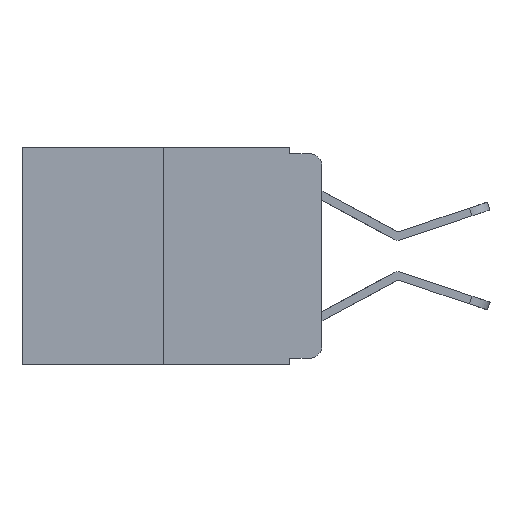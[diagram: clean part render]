
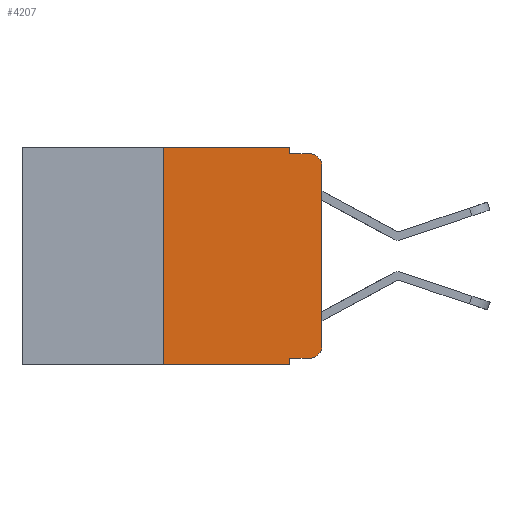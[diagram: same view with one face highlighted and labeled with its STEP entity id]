
A CAD part, left-side view. The second image highlights one B-rep face of the part: STEP entity #4207.
In plain terms, the highlighted planar face has unit normal (-1, 0, 0).
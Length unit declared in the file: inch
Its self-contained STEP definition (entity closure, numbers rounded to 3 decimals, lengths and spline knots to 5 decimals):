
#212 = LINE ( 'NONE', #8934, #7662 ) ;
#297 = EDGE_CURVE ( 'NONE', #12256, #12017, #4708, .T. ) ;
#333 = VERTEX_POINT ( 'NONE', #1383 ) ;
#402 = CARTESIAN_POINT ( 'NONE',  ( 0., 0.02, -0.01 ) ) ;
#581 = CARTESIAN_POINT ( 'NONE',  ( 0., 0.02, -0.313 ) ) ;
#636 = DIRECTION ( 'NONE',  ( 0., -1., 0. ) ) ;
#1046 = DIRECTION ( 'NONE',  ( 0., 0., 1. ) ) ;
#1383 = CARTESIAN_POINT ( 'NONE',  ( 0., 0., -0.03 ) ) ;
#1679 = EDGE_CURVE ( 'NONE', #333, #10944, #9235, .T. ) ;
#2024 = PLANE ( 'NONE',  #10068 ) ;
#2312 = CARTESIAN_POINT ( 'NONE',  ( 0., 0.051, -0.333 ) ) ;
#2978 = CARTESIAN_POINT ( 'NONE',  ( 0., 0.051, -0.01 ) ) ;
#3108 = EDGE_CURVE ( 'NONE', #14213, #8641, #9107, .T. ) ;
#3114 = ORIENTED_EDGE ( 'NONE', *, *, #12327, .T. ) ;
#3122 = DIRECTION ( 'NONE',  ( -1., 0., 0. ) ) ;
#3251 = FACE_OUTER_BOUND ( 'NONE', #3727, .T. ) ;
#3275 = DIRECTION ( 'NONE',  ( -1., 0., 0. ) ) ;
#3452 = DIRECTION ( 'NONE',  ( 0., 0., -1. ) ) ;
#3561 = CARTESIAN_POINT ( 'NONE',  ( 0., 0.051, 0. ) ) ;
#3665 = ORIENTED_EDGE ( 'NONE', *, *, #6255, .T. ) ;
#3727 = EDGE_LOOP ( 'NONE', ( #3665, #12600, #4536, #15587, #9954, #3835, #3114, #15372, #4014, #5535 ) ) ;
#3753 = VECTOR ( 'NONE', #6467, 39.37008 ) ;
#3756 = VECTOR ( 'NONE', #6733, 39.37008 ) ;
#3835 = ORIENTED_EDGE ( 'NONE', *, *, #9196, .F. ) ;
#4014 = ORIENTED_EDGE ( 'NONE', *, *, #7070, .T. ) ;
#4199 = CARTESIAN_POINT ( 'NONE',  ( 0., 0.051, -0.01 ) ) ;
#4207 = ADVANCED_FACE ( 'NONE', ( #3251 ), #2024, .F. ) ;
#4519 = DIRECTION ( 'NONE',  ( 0., 0., -1. ) ) ;
#4536 = ORIENTED_EDGE ( 'NONE', *, *, #13180, .F. ) ;
#4569 = VERTEX_POINT ( 'NONE', #14029 ) ;
#4619 = CARTESIAN_POINT ( 'NONE',  ( 0., 0.25, -0.343 ) ) ;
#4708 = LINE ( 'NONE', #14584, #7427 ) ;
#4967 = VERTEX_POINT ( 'NONE', #10466 ) ;
#5535 = ORIENTED_EDGE ( 'NONE', *, *, #10869, .T. ) ;
#5554 = CARTESIAN_POINT ( 'NONE',  ( 0., 0.473, 0. ) ) ;
#5562 = VECTOR ( 'NONE', #8640, 39.37008 ) ;
#6005 = CARTESIAN_POINT ( 'NONE',  ( 0., 0.473, -0.343 ) ) ;
#6115 = VECTOR ( 'NONE', #636, 39.37008 ) ;
#6255 = EDGE_CURVE ( 'NONE', #4569, #333, #212, .T. ) ;
#6301 = DIRECTION ( 'NONE',  ( 0., 0., -1. ) ) ;
#6404 = VECTOR ( 'NONE', #1046, 39.37008 ) ;
#6467 = DIRECTION ( 'NONE',  ( 0., -1., 0. ) ) ;
#6733 = DIRECTION ( 'NONE',  ( 0., -1., 0. ) ) ;
#7070 = EDGE_CURVE ( 'NONE', #12256, #4967, #12987, .T. ) ;
#7427 = VECTOR ( 'NONE', #3452, 39.37008 ) ;
#7662 = VECTOR ( 'NONE', #12722, 39.37008 ) ;
#8383 = LINE ( 'NONE', #6005, #5562 ) ;
#8492 = LINE ( 'NONE', #13249, #6404 ) ;
#8640 = DIRECTION ( 'NONE',  ( 0., -1., 0. ) ) ;
#8641 = VERTEX_POINT ( 'NONE', #12896 ) ;
#8934 = CARTESIAN_POINT ( 'NONE',  ( 0., 0., 0. ) ) ;
#9107 = LINE ( 'NONE', #12878, #3753 ) ;
#9196 = EDGE_CURVE ( 'NONE', #15084, #14213, #8492, .T. ) ;
#9235 = CIRCLE ( 'NONE', #10229, 0.02 ) ;
#9410 = CARTESIAN_POINT ( 'NONE',  ( 0., 0.02, -0.03 ) ) ;
#9634 = DIRECTION ( 'NONE',  ( 1., 0., 0. ) ) ;
#9954 = ORIENTED_EDGE ( 'NONE', *, *, #3108, .F. ) ;
#10068 = AXIS2_PLACEMENT_3D ( 'NONE', #5554, #9634, #10830 ) ;
#10219 = EDGE_CURVE ( 'NONE', #8641, #13550, #16103, .T. ) ;
#10229 = AXIS2_PLACEMENT_3D ( 'NONE', #9410, #3122, #15647 ) ;
#10466 = CARTESIAN_POINT ( 'NONE',  ( 0., 0.02, -0.333 ) ) ;
#10830 = DIRECTION ( 'NONE',  ( 0., 0., -1. ) ) ;
#10869 = EDGE_CURVE ( 'NONE', #4967, #4569, #15546, .T. ) ;
#10944 = VERTEX_POINT ( 'NONE', #402 ) ;
#11000 = CARTESIAN_POINT ( 'NONE',  ( 0., 0.25, 0. ) ) ;
#12017 = VERTEX_POINT ( 'NONE', #13523 ) ;
#12256 = VERTEX_POINT ( 'NONE', #14013 ) ;
#12327 = EDGE_CURVE ( 'NONE', #15084, #12017, #8383, .T. ) ;
#12600 = ORIENTED_EDGE ( 'NONE', *, *, #1679, .T. ) ;
#12657 = AXIS2_PLACEMENT_3D ( 'NONE', #581, #3275, #4519 ) ;
#12722 = DIRECTION ( 'NONE',  ( 0., 0., 1. ) ) ;
#12878 = CARTESIAN_POINT ( 'NONE',  ( 0., 0.473, 0. ) ) ;
#12896 = CARTESIAN_POINT ( 'NONE',  ( 0., 0.051, 0. ) ) ;
#12987 = LINE ( 'NONE', #2312, #6115 ) ;
#13180 = EDGE_CURVE ( 'NONE', #13550, #10944, #14115, .T. ) ;
#13249 = CARTESIAN_POINT ( 'NONE',  ( 0., 0.25, 0. ) ) ;
#13523 = CARTESIAN_POINT ( 'NONE',  ( 0., 0.051, -0.343 ) ) ;
#13550 = VERTEX_POINT ( 'NONE', #4199 ) ;
#14013 = CARTESIAN_POINT ( 'NONE',  ( 0., 0.051, -0.333 ) ) ;
#14029 = CARTESIAN_POINT ( 'NONE',  ( 0., 0., -0.313 ) ) ;
#14115 = LINE ( 'NONE', #2978, #3756 ) ;
#14213 = VERTEX_POINT ( 'NONE', #11000 ) ;
#14584 = CARTESIAN_POINT ( 'NONE',  ( 0., 0.051, 0. ) ) ;
#15084 = VERTEX_POINT ( 'NONE', #4619 ) ;
#15272 = VECTOR ( 'NONE', #6301, 39.37008 ) ;
#15372 = ORIENTED_EDGE ( 'NONE', *, *, #297, .F. ) ;
#15546 = CIRCLE ( 'NONE', #12657, 0.02 ) ;
#15587 = ORIENTED_EDGE ( 'NONE', *, *, #10219, .F. ) ;
#15647 = DIRECTION ( 'NONE',  ( 0., 0., -1. ) ) ;
#16103 = LINE ( 'NONE', #3561, #15272 ) ;
